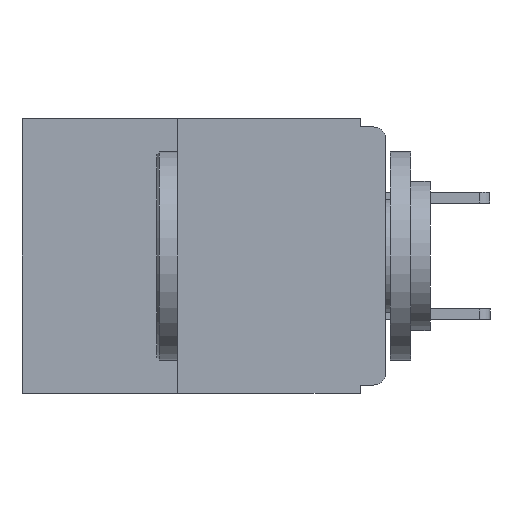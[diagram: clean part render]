
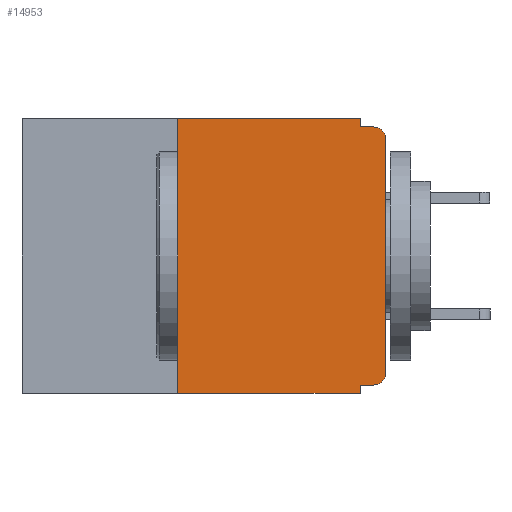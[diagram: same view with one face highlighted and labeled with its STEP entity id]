
A CAD part, left-side view. The second image highlights one B-rep face of the part: STEP entity #14953.
In plain terms, the highlighted planar face has unit normal (-1, 0, 0).
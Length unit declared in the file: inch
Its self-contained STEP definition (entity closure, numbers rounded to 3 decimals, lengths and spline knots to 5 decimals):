
#231 = AXIS2_PLACEMENT_3D ( 'NONE', #9365, #1204, #10740 ) ;
#645 = CARTESIAN_POINT ( 'NONE',  ( 0., 0.437, 0. ) ) ;
#691 = DIRECTION ( 'NONE',  ( 0., -1., 0. ) ) ;
#836 = EDGE_CURVE ( 'NONE', #1209, #7715, #12536, .T. ) ;
#894 = LINE ( 'NONE', #11648, #4629 ) ;
#916 = CARTESIAN_POINT ( 'NONE',  ( 0., 0.25, 0. ) ) ;
#1063 = ORIENTED_EDGE ( 'NONE', *, *, #1607, .F. ) ;
#1085 = AXIS2_PLACEMENT_3D ( 'NONE', #645, #6240, #15569 ) ;
#1204 = DIRECTION ( 'NONE',  ( -1., 0., 0. ) ) ;
#1209 = VERTEX_POINT ( 'NONE', #9648 ) ;
#1607 = EDGE_CURVE ( 'NONE', #1209, #5222, #9806, .T. ) ;
#1964 = EDGE_CURVE ( 'NONE', #2337, #5821, #14582, .T. ) ;
#2337 = VERTEX_POINT ( 'NONE', #17027 ) ;
#2561 = CARTESIAN_POINT ( 'NONE',  ( 0., 0.015, -0.01 ) ) ;
#3250 = EDGE_CURVE ( 'NONE', #5603, #7715, #9090, .T. ) ;
#3888 = CARTESIAN_POINT ( 'NONE',  ( 0., 0.031, -0.32 ) ) ;
#3902 = CARTESIAN_POINT ( 'NONE',  ( 0., 0.031, 0. ) ) ;
#4321 = CARTESIAN_POINT ( 'NONE',  ( 0., 0., -0.32 ) ) ;
#4629 = VECTOR ( 'NONE', #691, 39.37008 ) ;
#4697 = VERTEX_POINT ( 'NONE', #5714 ) ;
#5222 = VERTEX_POINT ( 'NONE', #916 ) ;
#5463 = VECTOR ( 'NONE', #7966, 39.37008 ) ;
#5603 = VERTEX_POINT ( 'NONE', #3888 ) ;
#5714 = CARTESIAN_POINT ( 'NONE',  ( 0., 0., -0.025 ) ) ;
#5821 = VERTEX_POINT ( 'NONE', #14088 ) ;
#6240 = DIRECTION ( 'NONE',  ( 1., 0., 0. ) ) ;
#6374 = VECTOR ( 'NONE', #15040, 39.37008 ) ;
#6889 = CARTESIAN_POINT ( 'NONE',  ( 0., 0.031, 0. ) ) ;
#7146 = DIRECTION ( 'NONE',  ( 0., 0., -1. ) ) ;
#7395 = EDGE_CURVE ( 'NONE', #5821, #4697, #8663, .T. ) ;
#7715 = VERTEX_POINT ( 'NONE', #10337 ) ;
#7966 = DIRECTION ( 'NONE',  ( 0., 0., -1. ) ) ;
#7978 = CARTESIAN_POINT ( 'NONE',  ( 0., 0., -0.01 ) ) ;
#8590 = EDGE_LOOP ( 'NONE', ( #10577, #12107, #14084, #17137, #11687, #1063, #8751, #12599, #10666, #12051 ) ) ;
#8663 = LINE ( 'NONE', #13831, #12680 ) ;
#8749 = VERTEX_POINT ( 'NONE', #10528 ) ;
#8751 = ORIENTED_EDGE ( 'NONE', *, *, #836, .T. ) ;
#8811 = EDGE_CURVE ( 'NONE', #8749, #12293, #16860, .T. ) ;
#8854 = FACE_OUTER_BOUND ( 'NONE', #8590, .T. ) ;
#8942 = VECTOR ( 'NONE', #15743, 39.37008 ) ;
#9090 = LINE ( 'NONE', #12500, #16523 ) ;
#9323 = EDGE_CURVE ( 'NONE', #15250, #8749, #16079, .T. ) ;
#9365 = CARTESIAN_POINT ( 'NONE',  ( 0., 0.015, -0.025 ) ) ;
#9373 = VECTOR ( 'NONE', #16433, 39.37008 ) ;
#9617 = CARTESIAN_POINT ( 'NONE',  ( 0., 0.015, -0.305 ) ) ;
#9648 = CARTESIAN_POINT ( 'NONE',  ( 0., 0.25, -0.33 ) ) ;
#9806 = LINE ( 'NONE', #12650, #9373 ) ;
#9957 = LINE ( 'NONE', #4321, #6374 ) ;
#10337 = CARTESIAN_POINT ( 'NONE',  ( 0., 0.031, -0.33 ) ) ;
#10502 = AXIS2_PLACEMENT_3D ( 'NONE', #9617, #10770, #7146 ) ;
#10528 = CARTESIAN_POINT ( 'NONE',  ( 0., 0.031, -0.01 ) ) ;
#10577 = ORIENTED_EDGE ( 'NONE', *, *, #7395, .T. ) ;
#10666 = ORIENTED_EDGE ( 'NONE', *, *, #14237, .F. ) ;
#10740 = DIRECTION ( 'NONE',  ( 0., 0., -1. ) ) ;
#10770 = DIRECTION ( 'NONE',  ( -1., 0., 0. ) ) ;
#10956 = CIRCLE ( 'NONE', #231, 0.015 ) ;
#11648 = CARTESIAN_POINT ( 'NONE',  ( 0., 0.437, 0. ) ) ;
#11687 = ORIENTED_EDGE ( 'NONE', *, *, #15578, .F. ) ;
#12051 = ORIENTED_EDGE ( 'NONE', *, *, #1964, .T. ) ;
#12107 = ORIENTED_EDGE ( 'NONE', *, *, #16291, .T. ) ;
#12293 = VERTEX_POINT ( 'NONE', #2561 ) ;
#12356 = DIRECTION ( 'NONE',  ( 0., 0., -1. ) ) ;
#12500 = CARTESIAN_POINT ( 'NONE',  ( 0., 0.031, -0.33 ) ) ;
#12536 = LINE ( 'NONE', #15507, #8942 ) ;
#12599 = ORIENTED_EDGE ( 'NONE', *, *, #3250, .F. ) ;
#12650 = CARTESIAN_POINT ( 'NONE',  ( 0., 0.25, -0.33 ) ) ;
#12680 = VECTOR ( 'NONE', #13793, 39.37008 ) ;
#13464 = VECTOR ( 'NONE', #17178, 39.37008 ) ;
#13793 = DIRECTION ( 'NONE',  ( 0., 0., 1. ) ) ;
#13831 = CARTESIAN_POINT ( 'NONE',  ( 0., 0., 0. ) ) ;
#14084 = ORIENTED_EDGE ( 'NONE', *, *, #8811, .F. ) ;
#14088 = CARTESIAN_POINT ( 'NONE',  ( 0., 0., -0.305 ) ) ;
#14237 = EDGE_CURVE ( 'NONE', #2337, #5603, #9957, .T. ) ;
#14269 = PLANE ( 'NONE',  #1085 ) ;
#14582 = CIRCLE ( 'NONE', #10502, 0.015 ) ;
#14953 = ADVANCED_FACE ( 'NONE', ( #8854 ), #14269, .F. ) ;
#15040 = DIRECTION ( 'NONE',  ( 0., 1., 0. ) ) ;
#15250 = VERTEX_POINT ( 'NONE', #6889 ) ;
#15507 = CARTESIAN_POINT ( 'NONE',  ( 0., 0.437, -0.33 ) ) ;
#15569 = DIRECTION ( 'NONE',  ( 0., 0., -1. ) ) ;
#15578 = EDGE_CURVE ( 'NONE', #5222, #15250, #894, .T. ) ;
#15743 = DIRECTION ( 'NONE',  ( 0., -1., 0. ) ) ;
#16079 = LINE ( 'NONE', #3902, #5463 ) ;
#16291 = EDGE_CURVE ( 'NONE', #4697, #12293, #10956, .T. ) ;
#16433 = DIRECTION ( 'NONE',  ( 0., 0., 1. ) ) ;
#16523 = VECTOR ( 'NONE', #12356, 39.37008 ) ;
#16860 = LINE ( 'NONE', #7978, #13464 ) ;
#17027 = CARTESIAN_POINT ( 'NONE',  ( 0., 0.015, -0.32 ) ) ;
#17137 = ORIENTED_EDGE ( 'NONE', *, *, #9323, .F. ) ;
#17178 = DIRECTION ( 'NONE',  ( 0., -1., 0. ) ) ;
